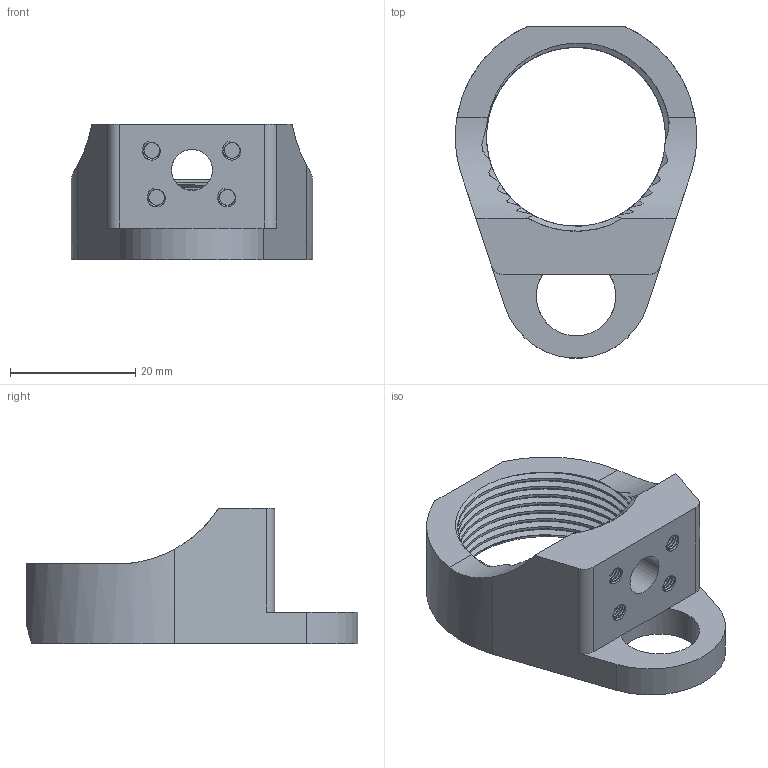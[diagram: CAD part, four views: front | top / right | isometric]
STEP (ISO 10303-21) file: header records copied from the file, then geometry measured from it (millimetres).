
FILE_DESCRIPTION(/* description */ (''),/* implementation_level */ '2;1');
FILE_NAME(/* name */ 'GG Buffer Tower v3.step',/* time_stamp */ '2024-01-16T15:52:36-05:00',/* author */ (''),/* organization */ (''),/* preprocessor_version */ 'ST-DEVELOPER v20',/* originating_system */ 'Autodesk Translation Framework v12.14.0.127',/* authorisation */ '');
FILE_SCHEMA (('AUTOMOTIVE_DESIGN { 1 0 10303 214 3 1 1 }'));
Length unit declared in the file: inch
Products named in the file (1): GG Buffer Tower
Bounding box: 38.51 x 52.94 x 21.67 mm (x, y, z)
Volume: 10868.9 mm3; surface area: 6676.3 mm2
Topology: 1 solids, 1 shells, 207 faces, 610 edges, 406 vertices
Faces by surface type: cylinder 163, bspline 28, plane 15, cone 1
Full cylindrical faces by diameter (mm): 2.529 x20, 3.086 x16, 6.553 x1, 12.7 x1, 28.555 x5, 30.162 x6
Entity records: 16159 total; most frequent: CARTESIAN_POINT 11449, ORIENTED_EDGE 1220, EDGE_CURVE 610, DIRECTION 599, B_SPLINE_CURVE_WITH_KNOTS 413, VERTEX_POINT 406, AXIS2_PLACEMENT_3D 222, EDGE_LOOP 214
